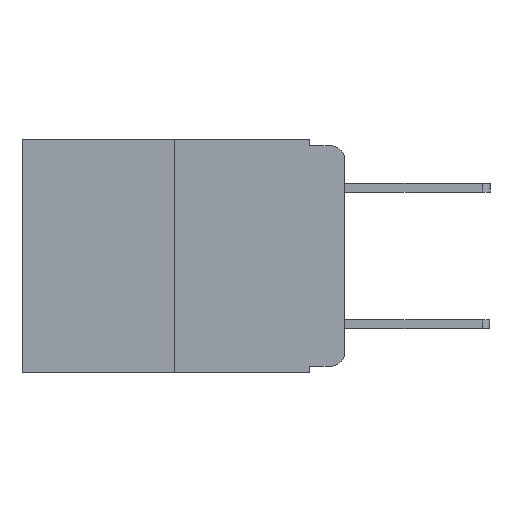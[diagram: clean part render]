
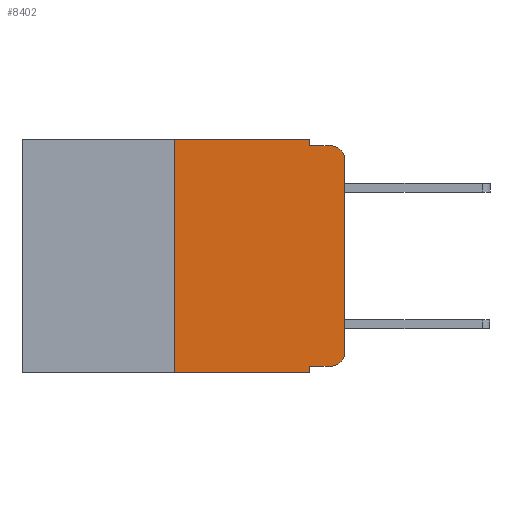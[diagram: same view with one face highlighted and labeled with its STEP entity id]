
A CAD part, left-side view. The second image highlights one B-rep face of the part: STEP entity #8402.
In plain terms, the highlighted planar face has unit normal (-1, 0, 0).
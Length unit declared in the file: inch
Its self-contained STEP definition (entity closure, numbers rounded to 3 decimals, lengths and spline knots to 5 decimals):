
#65 = EDGE_CURVE ( 'NONE', #992, #5626, #5305, .T. ) ;
#142 = PLANE ( 'NONE',  #1401 ) ;
#279 = DIRECTION ( 'NONE',  ( -1., 0., 0. ) ) ;
#319 = CARTESIAN_POINT ( 'NONE',  ( 0., 0.25, 0. ) ) ;
#410 = ORIENTED_EDGE ( 'NONE', *, *, #10947, .F. ) ;
#614 = AXIS2_PLACEMENT_3D ( 'NONE', #9443, #9453, #9552 ) ;
#667 = ORIENTED_EDGE ( 'NONE', *, *, #6247, .F. ) ;
#764 = EDGE_CURVE ( 'NONE', #2339, #7572, #953, .T. ) ;
#930 = ORIENTED_EDGE ( 'NONE', *, *, #1269, .F. ) ;
#953 = LINE ( 'NONE', #2192, #5724 ) ;
#992 = VERTEX_POINT ( 'NONE', #2321 ) ;
#1145 = CARTESIAN_POINT ( 'NONE',  ( 0., 0., -0.03 ) ) ;
#1176 = DIRECTION ( 'NONE',  ( 0., 0., -1. ) ) ;
#1242 = ORIENTED_EDGE ( 'NONE', *, *, #764, .F. ) ;
#1269 = EDGE_CURVE ( 'NONE', #10413, #2928, #4110, .T. ) ;
#1375 = VECTOR ( 'NONE', #3184, 39.37008 ) ;
#1401 = AXIS2_PLACEMENT_3D ( 'NONE', #5612, #6480, #1176 ) ;
#1402 = CARTESIAN_POINT ( 'NONE',  ( 0., 0.25, 0. ) ) ;
#1405 = ORIENTED_EDGE ( 'NONE', *, *, #4993, .T. ) ;
#1430 = CARTESIAN_POINT ( 'NONE',  ( 0., 0.051, -0.01 ) ) ;
#1777 = VECTOR ( 'NONE', #5941, 39.37008 ) ;
#1827 = LINE ( 'NONE', #3346, #6243 ) ;
#2179 = DIRECTION ( 'NONE',  ( 0., 0., -1. ) ) ;
#2192 = CARTESIAN_POINT ( 'NONE',  ( 0., 0.051, 0. ) ) ;
#2321 = CARTESIAN_POINT ( 'NONE',  ( 0., 0.02, -0.333 ) ) ;
#2339 = VERTEX_POINT ( 'NONE', #11391 ) ;
#2375 = FACE_OUTER_BOUND ( 'NONE', #6146, .T. ) ;
#2653 = ORIENTED_EDGE ( 'NONE', *, *, #4555, .T. ) ;
#2680 = CARTESIAN_POINT ( 'NONE',  ( 0., 0.051, -0.333 ) ) ;
#2791 = CIRCLE ( 'NONE', #5180, 0.02 ) ;
#2928 = VERTEX_POINT ( 'NONE', #1402 ) ;
#3028 = ORIENTED_EDGE ( 'NONE', *, *, #6587, .T. ) ;
#3033 = DIRECTION ( 'NONE',  ( 0., 0., 1. ) ) ;
#3184 = DIRECTION ( 'NONE',  ( 0., 0., -1. ) ) ;
#3345 = ORIENTED_EDGE ( 'NONE', *, *, #10117, .T. ) ;
#3346 = CARTESIAN_POINT ( 'NONE',  ( 0., 0.473, 0. ) ) ;
#3840 = VECTOR ( 'NONE', #3033, 39.37008 ) ;
#4110 = LINE ( 'NONE', #319, #3840 ) ;
#4111 = ORIENTED_EDGE ( 'NONE', *, *, #7932, .F. ) ;
#4117 = ORIENTED_EDGE ( 'NONE', *, *, #65, .T. ) ;
#4179 = CARTESIAN_POINT ( 'NONE',  ( 0., 0.051, -0.01 ) ) ;
#4458 = CARTESIAN_POINT ( 'NONE',  ( 0., 0.25, -0.343 ) ) ;
#4555 = EDGE_CURVE ( 'NONE', #5626, #8370, #6119, .T. ) ;
#4805 = CARTESIAN_POINT ( 'NONE',  ( 0., 0.051, -0.343 ) ) ;
#4992 = CARTESIAN_POINT ( 'NONE',  ( 0., 0., -0.313 ) ) ;
#4993 = EDGE_CURVE ( 'NONE', #10413, #7572, #8598, .T. ) ;
#5004 = CARTESIAN_POINT ( 'NONE',  ( 0., 0.02, -0.01 ) ) ;
#5180 = AXIS2_PLACEMENT_3D ( 'NONE', #5753, #279, #6593 ) ;
#5305 = CIRCLE ( 'NONE', #614, 0.02 ) ;
#5352 = DIRECTION ( 'NONE',  ( 0., -1., 0. ) ) ;
#5612 = CARTESIAN_POINT ( 'NONE',  ( 0., 0.473, 0. ) ) ;
#5626 = VERTEX_POINT ( 'NONE', #4992 ) ;
#5697 = LINE ( 'NONE', #2680, #7666 ) ;
#5724 = VECTOR ( 'NONE', #2179, 39.37008 ) ;
#5753 = CARTESIAN_POINT ( 'NONE',  ( 0., 0.02, -0.03 ) ) ;
#5941 = DIRECTION ( 'NONE',  ( 0., -1., 0. ) ) ;
#6038 = CARTESIAN_POINT ( 'NONE',  ( 0., 0., 0. ) ) ;
#6119 = LINE ( 'NONE', #6038, #10540 ) ;
#6146 = EDGE_LOOP ( 'NONE', ( #2653, #3345, #4111, #667, #410, #930, #1405, #1242, #3028, #4117 ) ) ;
#6243 = VECTOR ( 'NONE', #9255, 39.37008 ) ;
#6247 = EDGE_CURVE ( 'NONE', #8899, #10753, #10522, .T. ) ;
#6377 = VECTOR ( 'NONE', #10732, 39.37008 ) ;
#6480 = DIRECTION ( 'NONE',  ( 1., 0., 0. ) ) ;
#6571 = CARTESIAN_POINT ( 'NONE',  ( 0., 0.473, -0.343 ) ) ;
#6587 = EDGE_CURVE ( 'NONE', #2339, #992, #5697, .T. ) ;
#6593 = DIRECTION ( 'NONE',  ( 0., 0., -1. ) ) ;
#7066 = VERTEX_POINT ( 'NONE', #5004 ) ;
#7444 = CARTESIAN_POINT ( 'NONE',  ( 0., 0.051, 0. ) ) ;
#7572 = VERTEX_POINT ( 'NONE', #4805 ) ;
#7666 = VECTOR ( 'NONE', #5352, 39.37008 ) ;
#7932 = EDGE_CURVE ( 'NONE', #10753, #7066, #10896, .T. ) ;
#8370 = VERTEX_POINT ( 'NONE', #1145 ) ;
#8402 = ADVANCED_FACE ( 'NONE', ( #2375 ), #142, .F. ) ;
#8598 = LINE ( 'NONE', #6571, #6377 ) ;
#8899 = VERTEX_POINT ( 'NONE', #9440 ) ;
#9255 = DIRECTION ( 'NONE',  ( 0., -1., 0. ) ) ;
#9338 = DIRECTION ( 'NONE',  ( 0., 0., 1. ) ) ;
#9440 = CARTESIAN_POINT ( 'NONE',  ( 0., 0.051, 0. ) ) ;
#9443 = CARTESIAN_POINT ( 'NONE',  ( 0., 0.02, -0.313 ) ) ;
#9453 = DIRECTION ( 'NONE',  ( -1., 0., 0. ) ) ;
#9552 = DIRECTION ( 'NONE',  ( 0., 0., -1. ) ) ;
#10117 = EDGE_CURVE ( 'NONE', #8370, #7066, #2791, .T. ) ;
#10413 = VERTEX_POINT ( 'NONE', #4458 ) ;
#10522 = LINE ( 'NONE', #7444, #1375 ) ;
#10540 = VECTOR ( 'NONE', #9338, 39.37008 ) ;
#10732 = DIRECTION ( 'NONE',  ( 0., -1., 0. ) ) ;
#10753 = VERTEX_POINT ( 'NONE', #4179 ) ;
#10896 = LINE ( 'NONE', #1430, #1777 ) ;
#10947 = EDGE_CURVE ( 'NONE', #2928, #8899, #1827, .T. ) ;
#11391 = CARTESIAN_POINT ( 'NONE',  ( 0., 0.051, -0.333 ) ) ;
